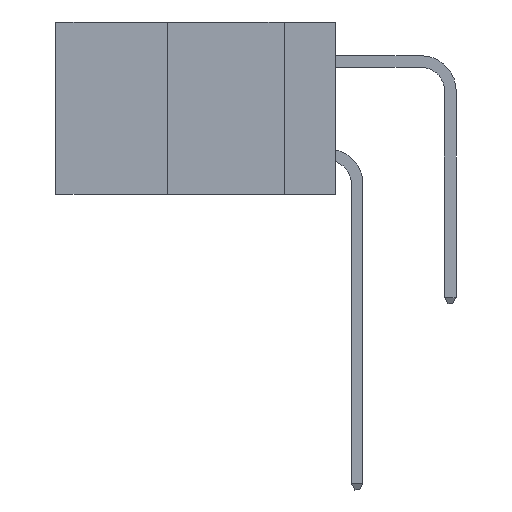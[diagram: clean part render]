
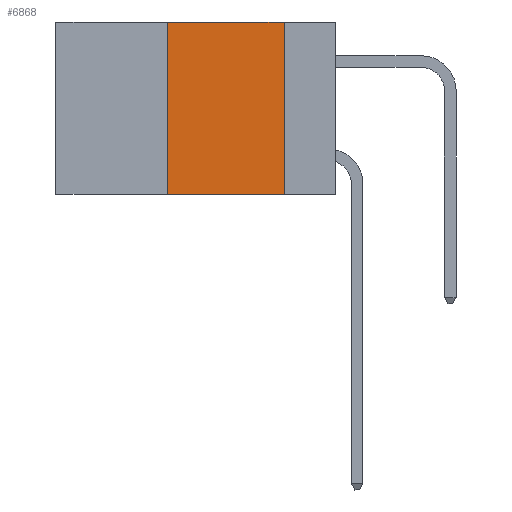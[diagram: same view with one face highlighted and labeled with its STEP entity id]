
A CAD part, left-side view. The second image highlights one B-rep face of the part: STEP entity #6868.
In plain terms, the highlighted planar face has unit normal (-1, 0, 0).
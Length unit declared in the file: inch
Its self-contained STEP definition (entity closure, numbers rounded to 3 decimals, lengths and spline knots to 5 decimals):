
#162 = ORIENTED_EDGE ( 'NONE', *, *, #13489, .T. ) ;
#368 = LINE ( 'NONE', #13008, #8224 ) ;
#558 = DIRECTION ( 'NONE',  ( 0., 0., -1. ) ) ;
#1460 = CARTESIAN_POINT ( 'NONE',  ( 0., 0.11, 0. ) ) ;
#2824 = CARTESIAN_POINT ( 'NONE',  ( 0., 0.11, 0. ) ) ;
#3584 = EDGE_CURVE ( 'NONE', #8666, #9533, #368, .T. ) ;
#3718 = VECTOR ( 'NONE', #8424, 39.37008 ) ;
#4389 = LINE ( 'NONE', #8488, #3718 ) ;
#4777 = VERTEX_POINT ( 'NONE', #5454 ) ;
#4882 = CARTESIAN_POINT ( 'NONE',  ( 0., 0.36, 0. ) ) ;
#5272 = ORIENTED_EDGE ( 'NONE', *, *, #3584, .F. ) ;
#5454 = CARTESIAN_POINT ( 'NONE',  ( 0., 0.11, -0.37 ) ) ;
#5554 = DIRECTION ( 'NONE',  ( 0., 0., -1. ) ) ;
#5633 = CARTESIAN_POINT ( 'NONE',  ( 0., 0.6, 0. ) ) ;
#6078 = EDGE_LOOP ( 'NONE', ( #9837, #9846, #5272, #162 ) ) ;
#6868 = ADVANCED_FACE ( 'NONE', ( #12076 ), #9083, .F. ) ;
#8177 = VECTOR ( 'NONE', #5554, 39.37008 ) ;
#8224 = VECTOR ( 'NONE', #9032, 39.37008 ) ;
#8246 = CARTESIAN_POINT ( 'NONE',  ( 0., 0.36, -0.37 ) ) ;
#8424 = DIRECTION ( 'NONE',  ( 0., -1., 0. ) ) ;
#8488 = CARTESIAN_POINT ( 'NONE',  ( 0., 0.6, 0. ) ) ;
#8666 = VERTEX_POINT ( 'NONE', #8246 ) ;
#8890 = LINE ( 'NONE', #13144, #13633 ) ;
#9032 = DIRECTION ( 'NONE',  ( 0., 0., 1. ) ) ;
#9083 = PLANE ( 'NONE',  #12507 ) ;
#9533 = VERTEX_POINT ( 'NONE', #4882 ) ;
#9689 = EDGE_CURVE ( 'NONE', #9533, #12780, #4389, .T. ) ;
#9774 = LINE ( 'NONE', #1460, #8177 ) ;
#9837 = ORIENTED_EDGE ( 'NONE', *, *, #10175, .F. ) ;
#9846 = ORIENTED_EDGE ( 'NONE', *, *, #9689, .F. ) ;
#10129 = DIRECTION ( 'NONE',  ( 1., 0., 0. ) ) ;
#10175 = EDGE_CURVE ( 'NONE', #12780, #4777, #9774, .T. ) ;
#11043 = DIRECTION ( 'NONE',  ( 0., -1., 0. ) ) ;
#12076 = FACE_OUTER_BOUND ( 'NONE', #6078, .T. ) ;
#12507 = AXIS2_PLACEMENT_3D ( 'NONE', #5633, #10129, #558 ) ;
#12780 = VERTEX_POINT ( 'NONE', #2824 ) ;
#13008 = CARTESIAN_POINT ( 'NONE',  ( 0., 0.36, 0. ) ) ;
#13144 = CARTESIAN_POINT ( 'NONE',  ( 0., 0.6, -0.37 ) ) ;
#13489 = EDGE_CURVE ( 'NONE', #8666, #4777, #8890, .T. ) ;
#13633 = VECTOR ( 'NONE', #11043, 39.37008 ) ;
